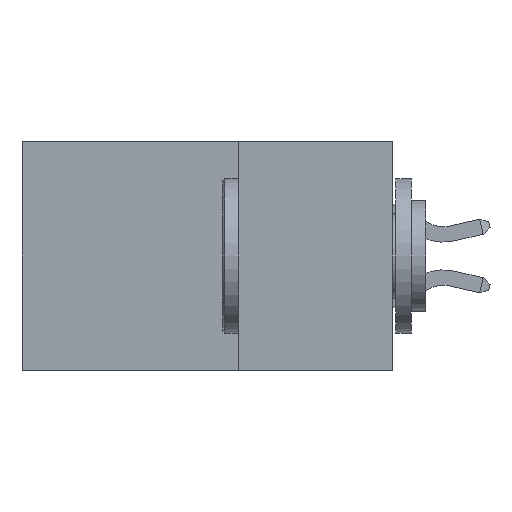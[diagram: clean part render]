
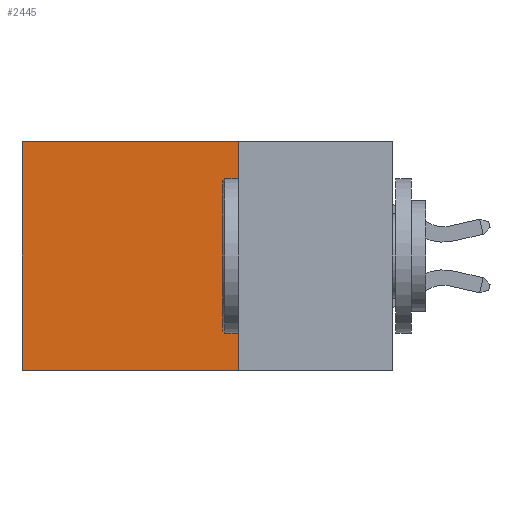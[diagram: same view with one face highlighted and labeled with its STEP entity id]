
A CAD part, left-side view. The second image highlights one B-rep face of the part: STEP entity #2445.
In plain terms, the highlighted planar face has unit normal (-1, 0, 0).
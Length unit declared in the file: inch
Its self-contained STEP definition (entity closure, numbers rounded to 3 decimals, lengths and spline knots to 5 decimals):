
#453 = EDGE_CURVE ( 'NONE', #2768, #12047, #4771, .T. ) ;
#514 = ORIENTED_EDGE ( 'NONE', *, *, #12036, .T. ) ;
#829 = CARTESIAN_POINT ( 'NONE',  ( 0.2875, 0.25, 0. ) ) ;
#847 = DIRECTION ( 'NONE',  ( 1., 0., 0. ) ) ;
#1070 = CARTESIAN_POINT ( 'NONE',  ( 0.2875, 0.25, -0.37 ) ) ;
#1258 = LINE ( 'NONE', #6283, #5717 ) ;
#1268 = LINE ( 'NONE', #8765, #9847 ) ;
#1672 = CARTESIAN_POINT ( 'NONE',  ( 0.2875, 0.6, 0. ) ) ;
#2293 = CARTESIAN_POINT ( 'NONE',  ( 0.2875, 0.25, -0.37 ) ) ;
#2445 = ADVANCED_FACE ( 'NONE', ( #6533 ), #13029, .F. ) ;
#2768 = VERTEX_POINT ( 'NONE', #9978 ) ;
#2793 = CARTESIAN_POINT ( 'NONE',  ( 0.2875, 0.6, -0.37 ) ) ;
#3784 = VERTEX_POINT ( 'NONE', #1070 ) ;
#4771 = LINE ( 'NONE', #829, #6936 ) ;
#5303 = VERTEX_POINT ( 'NONE', #2793 ) ;
#5717 = VECTOR ( 'NONE', #9308, 39.37008 ) ;
#6205 = DIRECTION ( 'NONE',  ( 0., 1., 0. ) ) ;
#6283 = CARTESIAN_POINT ( 'NONE',  ( 0.2875, 0.25, 0. ) ) ;
#6533 = FACE_OUTER_BOUND ( 'NONE', #6875, .T. ) ;
#6875 = EDGE_LOOP ( 'NONE', ( #514, #7163, #8462, #13605 ) ) ;
#6936 = VECTOR ( 'NONE', #6205, 39.37008 ) ;
#7163 = ORIENTED_EDGE ( 'NONE', *, *, #7637, .F. ) ;
#7256 = DIRECTION ( 'NONE',  ( 0., 0., -1. ) ) ;
#7637 = EDGE_CURVE ( 'NONE', #3784, #5303, #9411, .T. ) ;
#7813 = CARTESIAN_POINT ( 'NONE',  ( 0.2875, 0.25, 0. ) ) ;
#8283 = AXIS2_PLACEMENT_3D ( 'NONE', #7813, #847, #7256 ) ;
#8303 = VECTOR ( 'NONE', #9369, 39.37008 ) ;
#8462 = ORIENTED_EDGE ( 'NONE', *, *, #12282, .F. ) ;
#8765 = CARTESIAN_POINT ( 'NONE',  ( 0.2875, 0.6, 0. ) ) ;
#9308 = DIRECTION ( 'NONE',  ( 0., 0., -1. ) ) ;
#9369 = DIRECTION ( 'NONE',  ( 0., 1., 0. ) ) ;
#9411 = LINE ( 'NONE', #2293, #8303 ) ;
#9847 = VECTOR ( 'NONE', #13195, 39.37008 ) ;
#9978 = CARTESIAN_POINT ( 'NONE',  ( 0.2875, 0.25, 0. ) ) ;
#12036 = EDGE_CURVE ( 'NONE', #12047, #5303, #1268, .T. ) ;
#12047 = VERTEX_POINT ( 'NONE', #1672 ) ;
#12282 = EDGE_CURVE ( 'NONE', #2768, #3784, #1258, .T. ) ;
#13029 = PLANE ( 'NONE',  #8283 ) ;
#13195 = DIRECTION ( 'NONE',  ( 0., 0., -1. ) ) ;
#13605 = ORIENTED_EDGE ( 'NONE', *, *, #453, .T. ) ;
